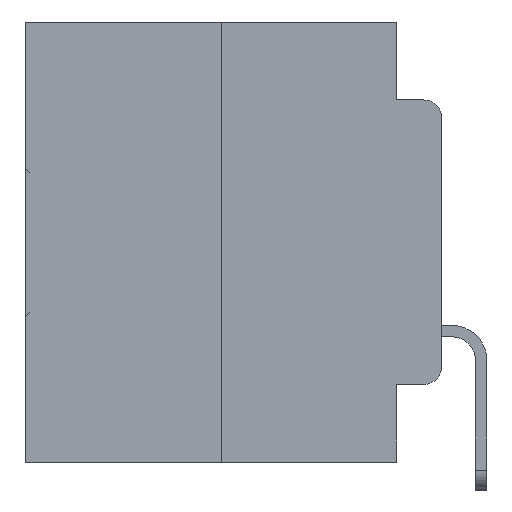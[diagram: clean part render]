
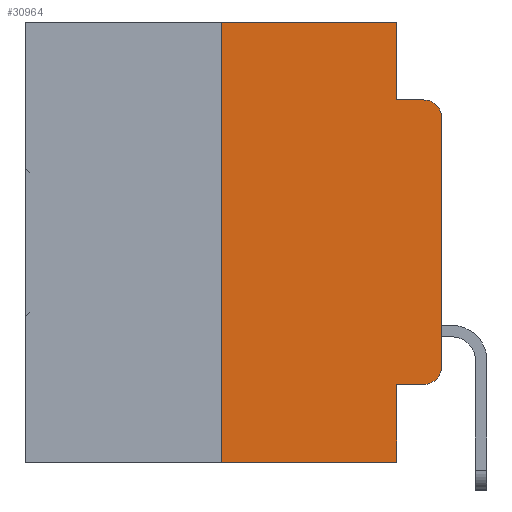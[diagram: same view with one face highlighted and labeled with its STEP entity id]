
A CAD part, left-side view. The second image highlights one B-rep face of the part: STEP entity #30964.
In plain terms, the highlighted planar face has unit normal (-1, 0, 0).
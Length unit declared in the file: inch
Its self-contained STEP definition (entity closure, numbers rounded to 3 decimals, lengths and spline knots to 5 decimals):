
#254 = DIRECTION ( 'NONE',  ( 0., 0., -1. ) ) ;
#1161 = EDGE_CURVE ( 'NONE', #5296, #20408, #5390, .T. ) ;
#1371 = EDGE_CURVE ( 'NONE', #16137, #5296, #29383, .T. ) ;
#1435 = CARTESIAN_POINT ( 'NONE',  ( 0., 0., 0. ) ) ;
#1506 = VERTEX_POINT ( 'NONE', #16299 ) ;
#1692 = ORIENTED_EDGE ( 'NONE', *, *, #9695, .F. ) ;
#2562 = VERTEX_POINT ( 'NONE', #30683 ) ;
#3924 = AXIS2_PLACEMENT_3D ( 'NONE', #8224, #15571, #254 ) ;
#4181 = DIRECTION ( 'NONE',  ( 0., 0., 1. ) ) ;
#4558 = VECTOR ( 'NONE', #4181, 39.37008 ) ;
#5099 = DIRECTION ( 'NONE',  ( 0., -1., 0. ) ) ;
#5296 = VERTEX_POINT ( 'NONE', #18204 ) ;
#5390 = LINE ( 'NONE', #1435, #4558 ) ;
#5434 = EDGE_CURVE ( 'NONE', #16690, #30900, #30122, .T. ) ;
#7753 = LINE ( 'NONE', #20760, #30423 ) ;
#7857 = CARTESIAN_POINT ( 'NONE',  ( 0., 0.02, -0.3915 ) ) ;
#8224 = CARTESIAN_POINT ( 'NONE',  ( 0., 0.473, 0. ) ) ;
#8654 = ORIENTED_EDGE ( 'NONE', *, *, #5434, .F. ) ;
#9187 = ORIENTED_EDGE ( 'NONE', *, *, #31511, .T. ) ;
#9501 = VECTOR ( 'NONE', #9991, 39.37008 ) ;
#9505 = LINE ( 'NONE', #10053, #22372 ) ;
#9695 = EDGE_CURVE ( 'NONE', #29140, #16690, #9505, .T. ) ;
#9991 = DIRECTION ( 'NONE',  ( 0., -1., 0. ) ) ;
#10053 = CARTESIAN_POINT ( 'NONE',  ( 0., 0.473, 0. ) ) ;
#10321 = DIRECTION ( 'NONE',  ( 0., 0., 1. ) ) ;
#10395 = DIRECTION ( 'NONE',  ( 0., 0., -1. ) ) ;
#10735 = PLANE ( 'NONE',  #3924 ) ;
#10808 = FACE_OUTER_BOUND ( 'NONE', #26894, .T. ) ;
#11272 = AXIS2_PLACEMENT_3D ( 'NONE', #13232, #30011, #15648 ) ;
#12500 = DIRECTION ( 'NONE',  ( 0., -1., 0. ) ) ;
#12937 = CARTESIAN_POINT ( 'NONE',  ( 0., 0.02, -0.4115 ) ) ;
#13232 = CARTESIAN_POINT ( 'NONE',  ( 0., 0.02, -0.1085 ) ) ;
#13309 = VERTEX_POINT ( 'NONE', #13819 ) ;
#13443 = EDGE_CURVE ( 'NONE', #13309, #16137, #23138, .T. ) ;
#13819 = CARTESIAN_POINT ( 'NONE',  ( 0., 0.051, -0.4115 ) ) ;
#13938 = DIRECTION ( 'NONE',  ( 0., 0., -1. ) ) ;
#14505 = EDGE_CURVE ( 'NONE', #17280, #1506, #7753, .T. ) ;
#15571 = DIRECTION ( 'NONE',  ( 1., 0., 0. ) ) ;
#15629 = ORIENTED_EDGE ( 'NONE', *, *, #13443, .T. ) ;
#15648 = DIRECTION ( 'NONE',  ( 0., 0., -1. ) ) ;
#15899 = AXIS2_PLACEMENT_3D ( 'NONE', #7857, #24812, #10395 ) ;
#16137 = VERTEX_POINT ( 'NONE', #12937 ) ;
#16299 = CARTESIAN_POINT ( 'NONE',  ( 0., 0.051, -0.5 ) ) ;
#16459 = CARTESIAN_POINT ( 'NONE',  ( 0., 0.051, 0. ) ) ;
#16690 = VERTEX_POINT ( 'NONE', #22810 ) ;
#16759 = ORIENTED_EDGE ( 'NONE', *, *, #22578, .F. ) ;
#17091 = EDGE_CURVE ( 'NONE', #30900, #2562, #23655, .T. ) ;
#17280 = VERTEX_POINT ( 'NONE', #18049 ) ;
#17407 = VECTOR ( 'NONE', #13938, 39.37008 ) ;
#17503 = CARTESIAN_POINT ( 'NONE',  ( 0., 0.051, -0.0885 ) ) ;
#18049 = CARTESIAN_POINT ( 'NONE',  ( 0., 0.25, -0.5 ) ) ;
#18130 = LINE ( 'NONE', #22387, #23763 ) ;
#18204 = CARTESIAN_POINT ( 'NONE',  ( 0., 0., -0.3915 ) ) ;
#20279 = CARTESIAN_POINT ( 'NONE',  ( 0., 0.051, -0.0885 ) ) ;
#20408 = VERTEX_POINT ( 'NONE', #28667 ) ;
#20562 = ORIENTED_EDGE ( 'NONE', *, *, #1161, .T. ) ;
#20596 = ORIENTED_EDGE ( 'NONE', *, *, #27937, .F. ) ;
#20760 = CARTESIAN_POINT ( 'NONE',  ( 0., 0.473, -0.5 ) ) ;
#20926 = CARTESIAN_POINT ( 'NONE',  ( 0., 0.25, 0. ) ) ;
#22372 = VECTOR ( 'NONE', #12500, 39.37008 ) ;
#22387 = CARTESIAN_POINT ( 'NONE',  ( 0., 0.25, 0. ) ) ;
#22578 = EDGE_CURVE ( 'NONE', #17280, #29140, #18130, .T. ) ;
#22810 = CARTESIAN_POINT ( 'NONE',  ( 0., 0.051, 0. ) ) ;
#23138 = LINE ( 'NONE', #31496, #9501 ) ;
#23168 = DIRECTION ( 'NONE',  ( 0., -1., 0. ) ) ;
#23570 = ORIENTED_EDGE ( 'NONE', *, *, #17091, .F. ) ;
#23599 = ORIENTED_EDGE ( 'NONE', *, *, #1371, .T. ) ;
#23655 = LINE ( 'NONE', #17503, #29193 ) ;
#23763 = VECTOR ( 'NONE', #10321, 39.37008 ) ;
#24138 = VECTOR ( 'NONE', #25871, 39.37008 ) ;
#24663 = ORIENTED_EDGE ( 'NONE', *, *, #14505, .T. ) ;
#24812 = DIRECTION ( 'NONE',  ( -1., 0., 0. ) ) ;
#24861 = LINE ( 'NONE', #30538, #24138 ) ;
#25871 = DIRECTION ( 'NONE',  ( 0., 0., -1. ) ) ;
#26894 = EDGE_LOOP ( 'NONE', ( #20562, #9187, #23570, #8654, #1692, #16759, #24663, #20596, #15629, #23599 ) ) ;
#27937 = EDGE_CURVE ( 'NONE', #13309, #1506, #24861, .T. ) ;
#28667 = CARTESIAN_POINT ( 'NONE',  ( 0., 0., -0.1085 ) ) ;
#29140 = VERTEX_POINT ( 'NONE', #20926 ) ;
#29171 = CIRCLE ( 'NONE', #11272, 0.02 ) ;
#29193 = VECTOR ( 'NONE', #5099, 39.37008 ) ;
#29383 = CIRCLE ( 'NONE', #15899, 0.02 ) ;
#30011 = DIRECTION ( 'NONE',  ( -1., 0., 0. ) ) ;
#30122 = LINE ( 'NONE', #16459, #17407 ) ;
#30423 = VECTOR ( 'NONE', #23168, 39.37008 ) ;
#30538 = CARTESIAN_POINT ( 'NONE',  ( 0., 0.051, 0. ) ) ;
#30683 = CARTESIAN_POINT ( 'NONE',  ( 0., 0.02, -0.0885 ) ) ;
#30900 = VERTEX_POINT ( 'NONE', #20279 ) ;
#30964 = ADVANCED_FACE ( 'NONE', ( #10808 ), #10735, .F. ) ;
#31496 = CARTESIAN_POINT ( 'NONE',  ( 0., 0.051, -0.4115 ) ) ;
#31511 = EDGE_CURVE ( 'NONE', #20408, #2562, #29171, .T. ) ;
